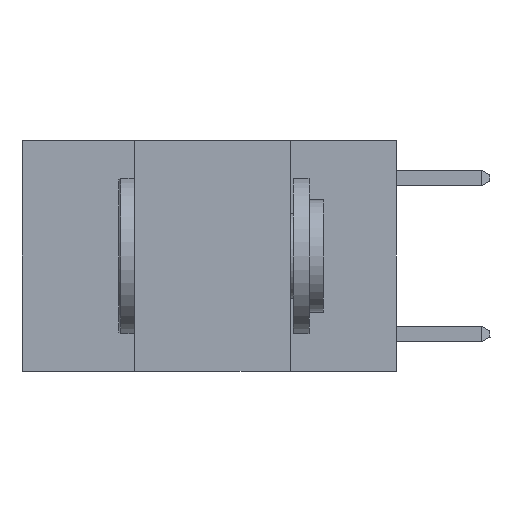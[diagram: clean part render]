
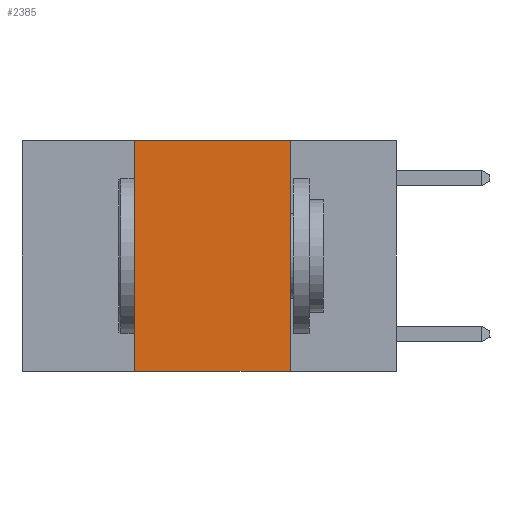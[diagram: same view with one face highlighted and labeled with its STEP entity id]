
A CAD part, left-side view. The second image highlights one B-rep face of the part: STEP entity #2385.
In plain terms, the highlighted planar face has unit normal (-1, 0, 0).
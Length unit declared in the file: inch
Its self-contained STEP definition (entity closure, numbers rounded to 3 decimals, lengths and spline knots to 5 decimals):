
#832 = CARTESIAN_POINT ( 'NONE',  ( 0., 0.6, -0.37 ) ) ;
#1508 = AXIS2_PLACEMENT_3D ( 'NONE', #10543, #13898, #6975 ) ;
#1529 = VERTEX_POINT ( 'NONE', #4666 ) ;
#1560 = EDGE_CURVE ( 'NONE', #1529, #3207, #4831, .T. ) ;
#1563 = ORIENTED_EDGE ( 'NONE', *, *, #10813, .T. ) ;
#2061 = CARTESIAN_POINT ( 'NONE',  ( 0., 0.17, 0. ) ) ;
#2385 = ADVANCED_FACE ( 'NONE', ( #9717 ), #12745, .F. ) ;
#2597 = DIRECTION ( 'NONE',  ( 0., 0., 1. ) ) ;
#2764 = CARTESIAN_POINT ( 'NONE',  ( 0., 0.42, 0. ) ) ;
#3207 = VERTEX_POINT ( 'NONE', #8465 ) ;
#3214 = EDGE_CURVE ( 'NONE', #5559, #5733, #7840, .T. ) ;
#3237 = EDGE_CURVE ( 'NONE', #3207, #5559, #13630, .T. ) ;
#3369 = DIRECTION ( 'NONE',  ( 0., -1., 0. ) ) ;
#3582 = CARTESIAN_POINT ( 'NONE',  ( 0., 0.17, 0. ) ) ;
#4595 = VECTOR ( 'NONE', #4860, 39.37008 ) ;
#4666 = CARTESIAN_POINT ( 'NONE',  ( 0., 0.42, -0.37 ) ) ;
#4831 = LINE ( 'NONE', #2764, #10869 ) ;
#4860 = DIRECTION ( 'NONE',  ( 0., 0., -1. ) ) ;
#5522 = ORIENTED_EDGE ( 'NONE', *, *, #3214, .F. ) ;
#5559 = VERTEX_POINT ( 'NONE', #2061 ) ;
#5733 = VERTEX_POINT ( 'NONE', #8398 ) ;
#6975 = DIRECTION ( 'NONE',  ( 0., 0., -1. ) ) ;
#7334 = CARTESIAN_POINT ( 'NONE',  ( 0., 0.6, 0. ) ) ;
#7840 = LINE ( 'NONE', #3582, #4595 ) ;
#8398 = CARTESIAN_POINT ( 'NONE',  ( 0., 0.17, -0.37 ) ) ;
#8465 = CARTESIAN_POINT ( 'NONE',  ( 0., 0.42, 0. ) ) ;
#9320 = VECTOR ( 'NONE', #3369, 39.37008 ) ;
#9717 = FACE_OUTER_BOUND ( 'NONE', #11769, .T. ) ;
#10543 = CARTESIAN_POINT ( 'NONE',  ( 0., 0.6, 0. ) ) ;
#10653 = VECTOR ( 'NONE', #10924, 39.37008 ) ;
#10813 = EDGE_CURVE ( 'NONE', #1529, #5733, #12398, .T. ) ;
#10869 = VECTOR ( 'NONE', #2597, 39.37008 ) ;
#10924 = DIRECTION ( 'NONE',  ( 0., -1., 0. ) ) ;
#11769 = EDGE_LOOP ( 'NONE', ( #5522, #12222, #12699, #1563 ) ) ;
#12222 = ORIENTED_EDGE ( 'NONE', *, *, #3237, .F. ) ;
#12398 = LINE ( 'NONE', #832, #9320 ) ;
#12699 = ORIENTED_EDGE ( 'NONE', *, *, #1560, .F. ) ;
#12745 = PLANE ( 'NONE',  #1508 ) ;
#13630 = LINE ( 'NONE', #7334, #10653 ) ;
#13898 = DIRECTION ( 'NONE',  ( 1., 0., 0. ) ) ;
